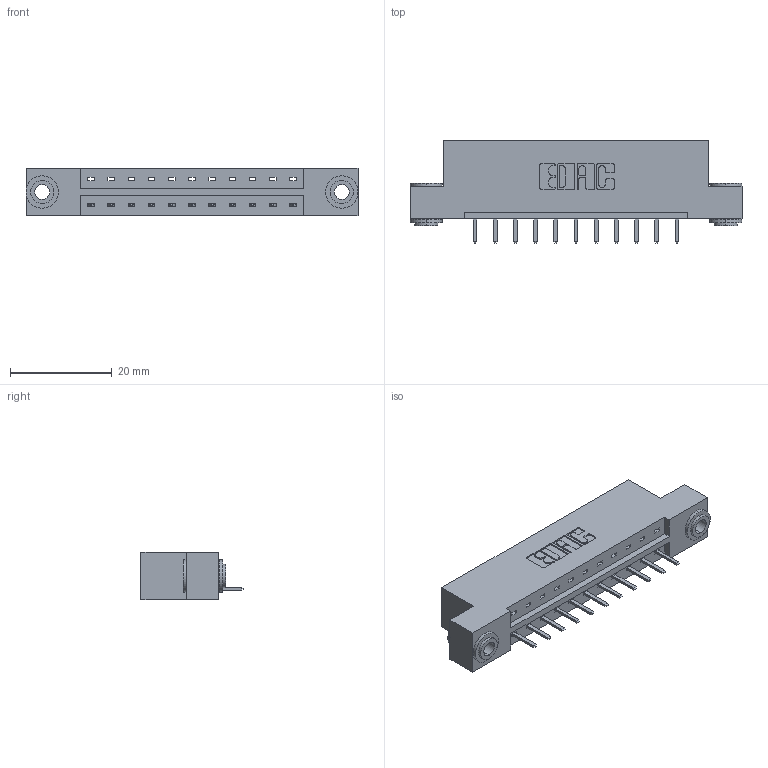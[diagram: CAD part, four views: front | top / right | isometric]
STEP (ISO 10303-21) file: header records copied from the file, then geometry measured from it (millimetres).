
FILE_DESCRIPTION (( 'STEP AP203' ), '1' );
FILE_NAME ('833-011-520-103.STEP', '2020-05-30T19:18:41', ( '' ), ( '' ), 'SwSTEP 2.0', 'SolidWorks 2020', '' );
FILE_SCHEMA (( 'CONFIG_CONTROL_DESIGN' ));
Length unit declared in the file: inch
Products named in the file (4): 345-250-002_345-250-002-102; 345-292-001_345-293-120; 833-011-520-103; 833 Part_Flush - .156 Dia - TH
Assembly tree (14 placements, depth 2):
  833-011-520-103
    833 Part_Flush - .156 Dia - TH
    345-292-001_345-293-120  x11
    345-250-002_345-250-002-102  x2
Bounding box: 65.13 x 20.02 x 9.4 mm (x, y, z)
Volume: 6274.6 mm3; surface area: 6702.7 mm2
Topology: 14 solids, 14 shells, 834 faces, 2411 edges, 1574 vertices
Faces by surface type: plane 564, cylinder 262, cone 8
Entity records: 11498 total; most frequent: CARTESIAN_POINT 1978, ORIENTED_EDGE 1906, DIRECTION 1753, EDGE_CURVE 953, LINE 797, VECTOR 797, VERTEX_POINT 630, AXIS2_PLACEMENT_3D 478
